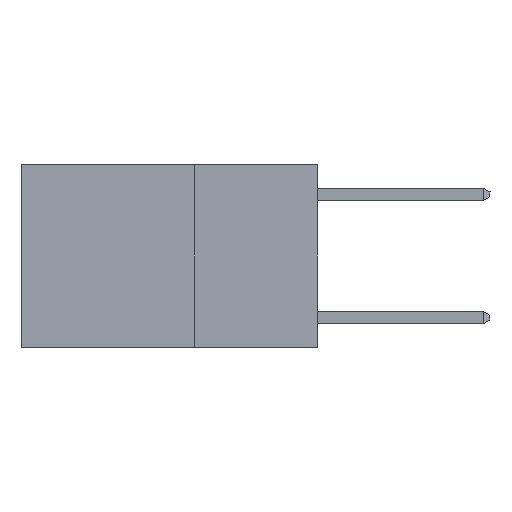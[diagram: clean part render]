
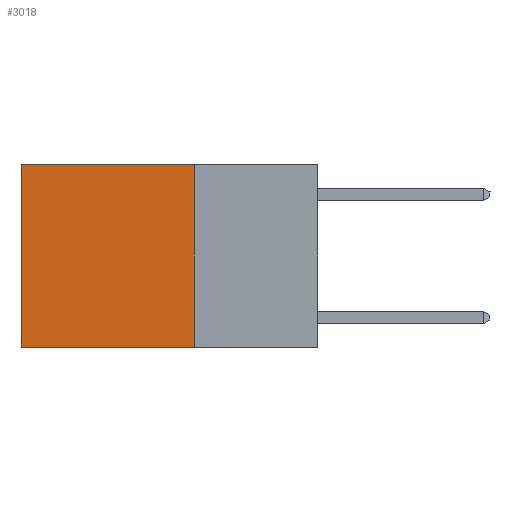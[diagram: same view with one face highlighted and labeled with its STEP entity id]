
A CAD part, left-side view. The second image highlights one B-rep face of the part: STEP entity #3018.
In plain terms, the highlighted planar face has unit normal (-1, 0, 0).
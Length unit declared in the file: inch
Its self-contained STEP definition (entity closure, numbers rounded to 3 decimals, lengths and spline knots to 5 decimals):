
#73 = VERTEX_POINT ( 'NONE', #607 ) ;
#280 = CARTESIAN_POINT ( 'NONE',  ( 0.2625, 0.25, 0. ) ) ;
#450 = VERTEX_POINT ( 'NONE', #12536 ) ;
#605 = VECTOR ( 'NONE', #7032, 39.37008 ) ;
#607 = CARTESIAN_POINT ( 'NONE',  ( 0.2625, 0.6, -0.37 ) ) ;
#1376 = VERTEX_POINT ( 'NONE', #6115 ) ;
#1529 = DIRECTION ( 'NONE',  ( 0., 0., -1. ) ) ;
#1578 = DIRECTION ( 'NONE',  ( 1., 0., 0. ) ) ;
#1599 = CARTESIAN_POINT ( 'NONE',  ( 0.2625, 0.25, 0. ) ) ;
#1638 = PLANE ( 'NONE',  #8359 ) ;
#1677 = VECTOR ( 'NONE', #1852, 39.37008 ) ;
#1706 = EDGE_CURVE ( 'NONE', #9588, #1376, #5191, .T. ) ;
#1852 = DIRECTION ( 'NONE',  ( 0., 0., -1. ) ) ;
#2551 = CARTESIAN_POINT ( 'NONE',  ( 0.2625, 0.25, 0. ) ) ;
#2597 = DIRECTION ( 'NONE',  ( 0., 0., -1. ) ) ;
#2991 = CARTESIAN_POINT ( 'NONE',  ( 0.2625, 0.25, 0. ) ) ;
#3018 = ADVANCED_FACE ( 'NONE', ( #7716 ), #1638, .F. ) ;
#3099 = DIRECTION ( 'NONE',  ( 0., 1., 0. ) ) ;
#4141 = VECTOR ( 'NONE', #2597, 39.37008 ) ;
#4888 = LINE ( 'NONE', #9747, #7455 ) ;
#4917 = EDGE_LOOP ( 'NONE', ( #6974, #6996, #7011, #7161 ) ) ;
#5191 = LINE ( 'NONE', #2551, #4141 ) ;
#6115 = CARTESIAN_POINT ( 'NONE',  ( 0.2625, 0.25, -0.37 ) ) ;
#6974 = ORIENTED_EDGE ( 'NONE', *, *, #14066, .T. ) ;
#6996 = ORIENTED_EDGE ( 'NONE', *, *, #7006, .F. ) ;
#7006 = EDGE_CURVE ( 'NONE', #1376, #73, #4888, .T. ) ;
#7011 = ORIENTED_EDGE ( 'NONE', *, *, #1706, .F. ) ;
#7032 = DIRECTION ( 'NONE',  ( 0., 1., 0. ) ) ;
#7161 = ORIENTED_EDGE ( 'NONE', *, *, #8092, .T. ) ;
#7455 = VECTOR ( 'NONE', #3099, 39.37008 ) ;
#7716 = FACE_OUTER_BOUND ( 'NONE', #4917, .T. ) ;
#7966 = LINE ( 'NONE', #9656, #1677 ) ;
#8092 = EDGE_CURVE ( 'NONE', #9588, #450, #11844, .T. ) ;
#8359 = AXIS2_PLACEMENT_3D ( 'NONE', #1599, #1578, #1529 ) ;
#9588 = VERTEX_POINT ( 'NONE', #2991 ) ;
#9656 = CARTESIAN_POINT ( 'NONE',  ( 0.2625, 0.6, 0. ) ) ;
#9747 = CARTESIAN_POINT ( 'NONE',  ( 0.2625, 0.25, -0.37 ) ) ;
#11844 = LINE ( 'NONE', #280, #605 ) ;
#12536 = CARTESIAN_POINT ( 'NONE',  ( 0.2625, 0.6, 0. ) ) ;
#14066 = EDGE_CURVE ( 'NONE', #450, #73, #7966, .T. ) ;
